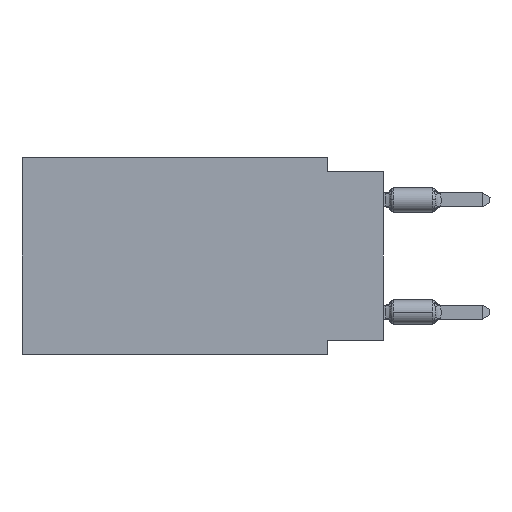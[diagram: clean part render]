
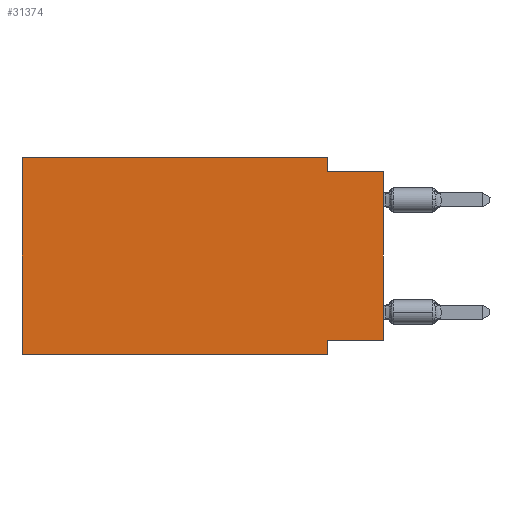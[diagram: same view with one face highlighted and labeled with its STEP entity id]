
A CAD part, left-side view. The second image highlights one B-rep face of the part: STEP entity #31374.
In plain terms, the highlighted planar face has unit normal (-1, 0, 0).
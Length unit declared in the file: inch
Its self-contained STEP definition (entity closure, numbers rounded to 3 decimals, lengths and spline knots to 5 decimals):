
#43 = CARTESIAN_POINT ( 'NONE',  ( 0., 0.645, 0. ) ) ;
#902 = ORIENTED_EDGE ( 'NONE', *, *, #31874, .F. ) ;
#2654 = VECTOR ( 'NONE', #25480, 39.37008 ) ;
#2700 = EDGE_CURVE ( 'NONE', #12776, #23364, #9412, .T. ) ;
#2779 = LINE ( 'NONE', #20358, #36338 ) ;
#4063 = DIRECTION ( 'NONE',  ( 0., -1., 0. ) ) ;
#4248 = CARTESIAN_POINT ( 'NONE',  ( 0., 0., -0.025 ) ) ;
#4937 = ORIENTED_EDGE ( 'NONE', *, *, #2700, .F. ) ;
#4958 = EDGE_CURVE ( 'NONE', #19361, #23238, #32748, .T. ) ;
#6671 = CARTESIAN_POINT ( 'NONE',  ( 0., 0.1, -0.325 ) ) ;
#6972 = CARTESIAN_POINT ( 'NONE',  ( 0., 0., -0.325 ) ) ;
#7197 = ORIENTED_EDGE ( 'NONE', *, *, #10730, .T. ) ;
#7682 = DIRECTION ( 'NONE',  ( 0., -1., 0. ) ) ;
#8615 = LINE ( 'NONE', #23185, #9421 ) ;
#9412 = LINE ( 'NONE', #31935, #18954 ) ;
#9421 = VECTOR ( 'NONE', #14864, 39.37008 ) ;
#9708 = CARTESIAN_POINT ( 'NONE',  ( 0., 0.645, 0. ) ) ;
#10515 = LINE ( 'NONE', #13357, #35281 ) ;
#10730 = EDGE_CURVE ( 'NONE', #28833, #20656, #10515, .T. ) ;
#12426 = VECTOR ( 'NONE', #29102, 39.37008 ) ;
#12471 = LINE ( 'NONE', #20610, #12426 ) ;
#12776 = VERTEX_POINT ( 'NONE', #6972 ) ;
#13357 = CARTESIAN_POINT ( 'NONE',  ( 0., 0.645, -0.35 ) ) ;
#14005 = FACE_OUTER_BOUND ( 'NONE', #22255, .T. ) ;
#14147 = CARTESIAN_POINT ( 'NONE',  ( 0., 0.645, 0. ) ) ;
#14864 = DIRECTION ( 'NONE',  ( 0., 0., -1. ) ) ;
#15437 = ORIENTED_EDGE ( 'NONE', *, *, #37006, .T. ) ;
#16189 = CARTESIAN_POINT ( 'NONE',  ( 0., 0.1, -0.35 ) ) ;
#18954 = VECTOR ( 'NONE', #23614, 39.37008 ) ;
#19361 = VERTEX_POINT ( 'NONE', #27482 ) ;
#19994 = ORIENTED_EDGE ( 'NONE', *, *, #35854, .F. ) ;
#20006 = LINE ( 'NONE', #14147, #2654 ) ;
#20245 = DIRECTION ( 'NONE',  ( 0., 0., -1. ) ) ;
#20358 = CARTESIAN_POINT ( 'NONE',  ( 0., 0., 0. ) ) ;
#20525 = LINE ( 'NONE', #9708, #27566 ) ;
#20610 = CARTESIAN_POINT ( 'NONE',  ( 0., 0.1, -0.35 ) ) ;
#20656 = VERTEX_POINT ( 'NONE', #16189 ) ;
#22255 = EDGE_LOOP ( 'NONE', ( #15437, #25904, #19994, #902, #37209, #7197, #23996, #4937 ) ) ;
#22957 = CARTESIAN_POINT ( 'NONE',  ( 0., 0., -0.025 ) ) ;
#23185 = CARTESIAN_POINT ( 'NONE',  ( 0., 0.1, 0. ) ) ;
#23238 = VERTEX_POINT ( 'NONE', #22957 ) ;
#23364 = VERTEX_POINT ( 'NONE', #6671 ) ;
#23614 = DIRECTION ( 'NONE',  ( 0., 1., 0. ) ) ;
#23996 = ORIENTED_EDGE ( 'NONE', *, *, #30242, .F. ) ;
#24051 = VERTEX_POINT ( 'NONE', #30287 ) ;
#24959 = CARTESIAN_POINT ( 'NONE',  ( 0., 0.645, 0. ) ) ;
#25005 = EDGE_CURVE ( 'NONE', #28833, #33551, #20525, .T. ) ;
#25480 = DIRECTION ( 'NONE',  ( 0., -1., 0. ) ) ;
#25524 = DIRECTION ( 'NONE',  ( 1., 0., 0. ) ) ;
#25904 = ORIENTED_EDGE ( 'NONE', *, *, #4958, .F. ) ;
#25933 = PLANE ( 'NONE',  #31605 ) ;
#26198 = DIRECTION ( 'NONE',  ( 0., 0., 1. ) ) ;
#26333 = VECTOR ( 'NONE', #4063, 39.37008 ) ;
#27482 = CARTESIAN_POINT ( 'NONE',  ( 0., 0.1, -0.025 ) ) ;
#27566 = VECTOR ( 'NONE', #32037, 39.37008 ) ;
#28833 = VERTEX_POINT ( 'NONE', #32388 ) ;
#29102 = DIRECTION ( 'NONE',  ( 0., 0., -1. ) ) ;
#30242 = EDGE_CURVE ( 'NONE', #23364, #20656, #12471, .T. ) ;
#30287 = CARTESIAN_POINT ( 'NONE',  ( 0., 0.1, 0. ) ) ;
#31374 = ADVANCED_FACE ( 'NONE', ( #14005 ), #25933, .F. ) ;
#31605 = AXIS2_PLACEMENT_3D ( 'NONE', #43, #25524, #20245 ) ;
#31874 = EDGE_CURVE ( 'NONE', #33551, #24051, #20006, .T. ) ;
#31935 = CARTESIAN_POINT ( 'NONE',  ( 0., 0., -0.325 ) ) ;
#32037 = DIRECTION ( 'NONE',  ( 0., 0., 1. ) ) ;
#32388 = CARTESIAN_POINT ( 'NONE',  ( 0., 0.645, -0.35 ) ) ;
#32748 = LINE ( 'NONE', #4248, #26333 ) ;
#33551 = VERTEX_POINT ( 'NONE', #24959 ) ;
#35281 = VECTOR ( 'NONE', #7682, 39.37008 ) ;
#35854 = EDGE_CURVE ( 'NONE', #24051, #19361, #8615, .T. ) ;
#36338 = VECTOR ( 'NONE', #26198, 39.37008 ) ;
#37006 = EDGE_CURVE ( 'NONE', #12776, #23238, #2779, .T. ) ;
#37209 = ORIENTED_EDGE ( 'NONE', *, *, #25005, .F. ) ;
